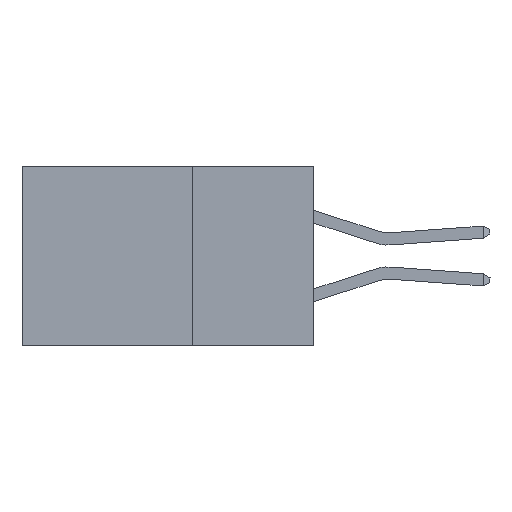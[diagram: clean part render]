
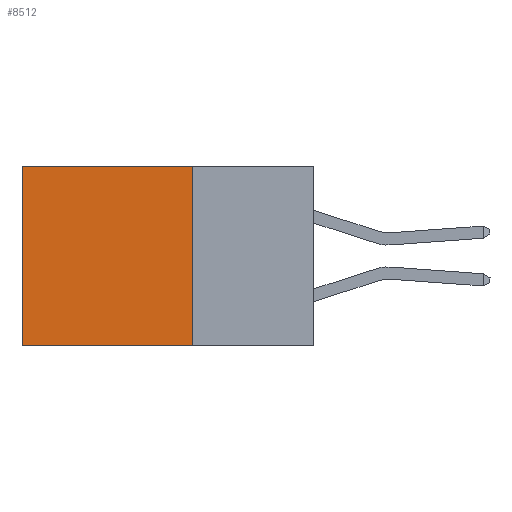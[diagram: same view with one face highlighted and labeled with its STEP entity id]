
A CAD part, left-side view. The second image highlights one B-rep face of the part: STEP entity #8512.
In plain terms, the highlighted planar face has unit normal (-1, 0, 0).
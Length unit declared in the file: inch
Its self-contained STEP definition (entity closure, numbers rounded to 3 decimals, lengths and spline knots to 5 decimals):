
#106 = CARTESIAN_POINT ( 'NONE',  ( 0.2875, 0.25, 0. ) ) ;
#661 = LINE ( 'NONE', #14601, #29544 ) ;
#2523 = ORIENTED_EDGE ( 'NONE', *, *, #4894, .F. ) ;
#4422 = EDGE_CURVE ( 'NONE', #10024, #10328, #14279, .T. ) ;
#4786 = CARTESIAN_POINT ( 'NONE',  ( 0.2875, 0.25, 0. ) ) ;
#4894 = EDGE_CURVE ( 'NONE', #26759, #19999, #25100, .T. ) ;
#4964 = AXIS2_PLACEMENT_3D ( 'NONE', #106, #17392, #28720 ) ;
#4993 = CARTESIAN_POINT ( 'NONE',  ( 0.2875, 0.6, -0.37 ) ) ;
#5498 = DIRECTION ( 'NONE',  ( 0., 1., 0. ) ) ;
#7953 = ORIENTED_EDGE ( 'NONE', *, *, #30086, .T. ) ;
#8512 = ADVANCED_FACE ( 'NONE', ( #9295 ), #11738, .F. ) ;
#9295 = FACE_OUTER_BOUND ( 'NONE', #23432, .T. ) ;
#9363 = CARTESIAN_POINT ( 'NONE',  ( 0.2875, 0.6, 0. ) ) ;
#9541 = DIRECTION ( 'NONE',  ( 0., 0., -1. ) ) ;
#9974 = ORIENTED_EDGE ( 'NONE', *, *, #16513, .F. ) ;
#10024 = VERTEX_POINT ( 'NONE', #16884 ) ;
#10328 = VERTEX_POINT ( 'NONE', #9363 ) ;
#11738 = PLANE ( 'NONE',  #4964 ) ;
#12488 = ORIENTED_EDGE ( 'NONE', *, *, #4422, .T. ) ;
#14279 = LINE ( 'NONE', #4786, #21376 ) ;
#14601 = CARTESIAN_POINT ( 'NONE',  ( 0.2875, 0.6, 0. ) ) ;
#14818 = CARTESIAN_POINT ( 'NONE',  ( 0.2875, 0.25, -0.37 ) ) ;
#16496 = LINE ( 'NONE', #28281, #26094 ) ;
#16513 = EDGE_CURVE ( 'NONE', #10024, #26759, #16496, .T. ) ;
#16884 = CARTESIAN_POINT ( 'NONE',  ( 0.2875, 0.25, 0. ) ) ;
#16955 = DIRECTION ( 'NONE',  ( 0., 0., -1. ) ) ;
#17392 = DIRECTION ( 'NONE',  ( 1., 0., 0. ) ) ;
#19542 = CARTESIAN_POINT ( 'NONE',  ( 0.2875, 0.25, -0.37 ) ) ;
#19999 = VERTEX_POINT ( 'NONE', #4993 ) ;
#21376 = VECTOR ( 'NONE', #25586, 39.37008 ) ;
#23432 = EDGE_LOOP ( 'NONE', ( #7953, #2523, #9974, #12488 ) ) ;
#25100 = LINE ( 'NONE', #19542, #26808 ) ;
#25586 = DIRECTION ( 'NONE',  ( 0., 1., 0. ) ) ;
#26094 = VECTOR ( 'NONE', #16955, 39.37008 ) ;
#26759 = VERTEX_POINT ( 'NONE', #14818 ) ;
#26808 = VECTOR ( 'NONE', #5498, 39.37008 ) ;
#28281 = CARTESIAN_POINT ( 'NONE',  ( 0.2875, 0.25, 0. ) ) ;
#28720 = DIRECTION ( 'NONE',  ( 0., 0., -1. ) ) ;
#29544 = VECTOR ( 'NONE', #9541, 39.37008 ) ;
#30086 = EDGE_CURVE ( 'NONE', #10328, #19999, #661, .T. ) ;
